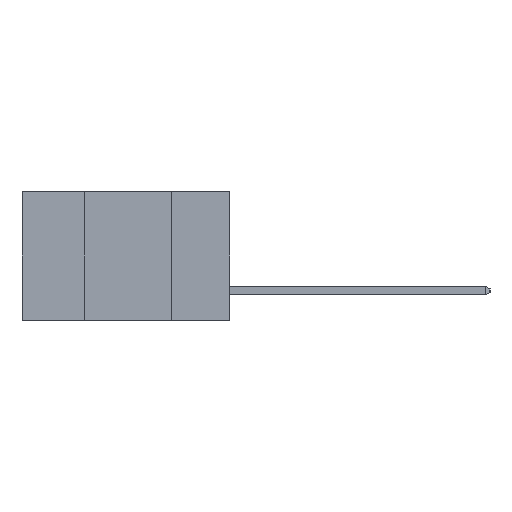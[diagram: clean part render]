
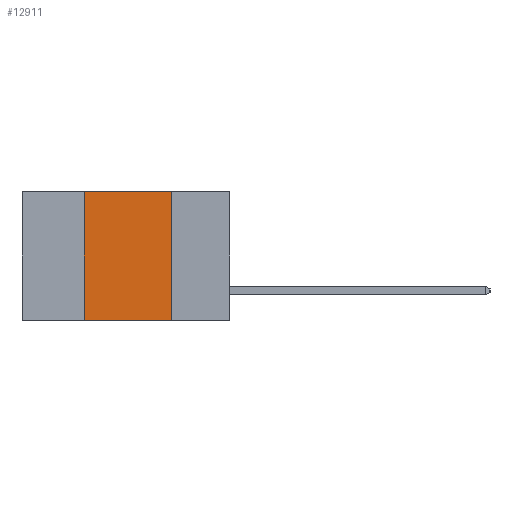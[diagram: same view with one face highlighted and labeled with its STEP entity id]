
A CAD part, left-side view. The second image highlights one B-rep face of the part: STEP entity #12911.
In plain terms, the highlighted planar face has unit normal (-1, 0, 0).
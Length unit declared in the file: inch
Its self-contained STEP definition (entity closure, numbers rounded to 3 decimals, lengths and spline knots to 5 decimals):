
#568 = ORIENTED_EDGE ( 'NONE', *, *, #13770, .F. ) ;
#1525 = ORIENTED_EDGE ( 'NONE', *, *, #11019, .F. ) ;
#3387 = CARTESIAN_POINT ( 'NONE',  ( 0., 0.17, -0.37 ) ) ;
#3513 = DIRECTION ( 'NONE',  ( 0., 0., -1. ) ) ;
#3749 = VECTOR ( 'NONE', #7636, 39.37008 ) ;
#3766 = VERTEX_POINT ( 'NONE', #11926 ) ;
#4203 = LINE ( 'NONE', #14520, #3749 ) ;
#5885 = EDGE_LOOP ( 'NONE', ( #1525, #568, #15224, #7418 ) ) ;
#6682 = VERTEX_POINT ( 'NONE', #15777 ) ;
#7016 = FACE_OUTER_BOUND ( 'NONE', #5885, .T. ) ;
#7418 = ORIENTED_EDGE ( 'NONE', *, *, #16934, .T. ) ;
#7453 = DIRECTION ( 'NONE',  ( 0., -1., 0. ) ) ;
#7458 = LINE ( 'NONE', #7521, #17504 ) ;
#7521 = CARTESIAN_POINT ( 'NONE',  ( 0., 0.6, 0. ) ) ;
#7636 = DIRECTION ( 'NONE',  ( 0., -1., 0. ) ) ;
#8236 = LINE ( 'NONE', #3387, #15572 ) ;
#9024 = AXIS2_PLACEMENT_3D ( 'NONE', #15082, #15039, #15020 ) ;
#11019 = EDGE_CURVE ( 'NONE', #3766, #6682, #8236, .T. ) ;
#11926 = CARTESIAN_POINT ( 'NONE',  ( 0., 0.17, 0. ) ) ;
#12258 = CARTESIAN_POINT ( 'NONE',  ( 0., 0.42, 0. ) ) ;
#12525 = VECTOR ( 'NONE', #15831, 39.37008 ) ;
#12911 = ADVANCED_FACE ( 'NONE', ( #7016 ), #15172, .F. ) ;
#13770 = EDGE_CURVE ( 'NONE', #17119, #3766, #7458, .T. ) ;
#14520 = CARTESIAN_POINT ( 'NONE',  ( 0., 0.6, -0.37 ) ) ;
#14619 = CARTESIAN_POINT ( 'NONE',  ( 0., 0.42, -0.37 ) ) ;
#14702 = EDGE_CURVE ( 'NONE', #14735, #17119, #16565, .T. ) ;
#14735 = VERTEX_POINT ( 'NONE', #14619 ) ;
#15020 = DIRECTION ( 'NONE',  ( 0., 0., -1. ) ) ;
#15039 = DIRECTION ( 'NONE',  ( 1., 0., 0. ) ) ;
#15082 = CARTESIAN_POINT ( 'NONE',  ( 0., 0.6, 0. ) ) ;
#15155 = CARTESIAN_POINT ( 'NONE',  ( 0., 0.42, -0.37 ) ) ;
#15172 = PLANE ( 'NONE',  #9024 ) ;
#15224 = ORIENTED_EDGE ( 'NONE', *, *, #14702, .F. ) ;
#15572 = VECTOR ( 'NONE', #3513, 39.37008 ) ;
#15777 = CARTESIAN_POINT ( 'NONE',  ( 0., 0.17, -0.37 ) ) ;
#15831 = DIRECTION ( 'NONE',  ( 0., 0., 1. ) ) ;
#16565 = LINE ( 'NONE', #15155, #12525 ) ;
#16934 = EDGE_CURVE ( 'NONE', #14735, #6682, #4203, .T. ) ;
#17119 = VERTEX_POINT ( 'NONE', #12258 ) ;
#17504 = VECTOR ( 'NONE', #7453, 39.37008 ) ;
